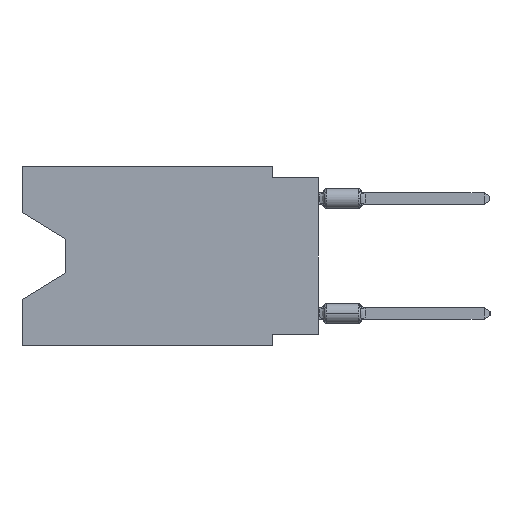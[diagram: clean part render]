
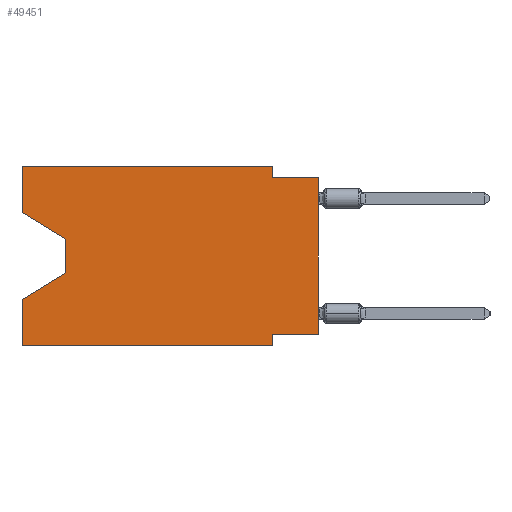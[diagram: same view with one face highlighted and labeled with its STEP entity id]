
A CAD part, left-side view. The second image highlights one B-rep face of the part: STEP entity #49451.
In plain terms, the highlighted planar face has unit normal (-1, 0, 0).
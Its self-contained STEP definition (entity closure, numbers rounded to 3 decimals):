
#1609 = DIRECTION ( 'NONE',  ( 0., -1., 0. ) ) ;
#1917 = LINE ( 'NONE', #22555, #45063 ) ;
#2264 = CARTESIAN_POINT ( 'NONE',  ( 0., 0., -9.271 ) ) ;
#2324 = VECTOR ( 'NONE', #37211, 1000. ) ;
#4034 = CARTESIAN_POINT ( 'NONE',  ( 0., 16.383, 0. ) ) ;
#5596 = VERTEX_POINT ( 'NONE', #2264 ) ;
#6420 = DIRECTION ( 'NONE',  ( 0., 0., -1. ) ) ;
#6921 = EDGE_CURVE ( 'NONE', #15326, #23665, #8161, .T. ) ;
#7123 = LINE ( 'NONE', #8091, #17892 ) ;
#7462 = ORIENTED_EDGE ( 'NONE', *, *, #47942, .T. ) ;
#7670 = EDGE_CURVE ( 'NONE', #15326, #26394, #16879, .T. ) ;
#8091 = CARTESIAN_POINT ( 'NONE',  ( 0., 16.383, -9.906 ) ) ;
#8161 = LINE ( 'NONE', #62636, #9732 ) ;
#8905 = CARTESIAN_POINT ( 'NONE',  ( 0., 16.383, -9.906 ) ) ;
#9318 = CARTESIAN_POINT ( 'NONE',  ( 0., 2.54, 0. ) ) ;
#9732 = VECTOR ( 'NONE', #18971, 1000. ) ;
#10109 = EDGE_CURVE ( 'NONE', #23665, #26422, #49308, .T. ) ;
#11025 = DIRECTION ( 'NONE',  ( 0., -0.855, -0.519 ) ) ;
#11275 = CARTESIAN_POINT ( 'NONE',  ( 0., 16.383, 0. ) ) ;
#11359 = DIRECTION ( 'NONE',  ( 1., 0., 0. ) ) ;
#12468 = LINE ( 'NONE', #52489, #16515 ) ;
#13906 = ORIENTED_EDGE ( 'NONE', *, *, #59940, .T. ) ;
#14040 = ORIENTED_EDGE ( 'NONE', *, *, #25743, .F. ) ;
#15326 = VERTEX_POINT ( 'NONE', #31941 ) ;
#15770 = LINE ( 'NONE', #35784, #16119 ) ;
#16119 = VECTOR ( 'NONE', #24974, 1000. ) ;
#16515 = VECTOR ( 'NONE', #46615, 1000. ) ;
#16879 = LINE ( 'NONE', #40542, #45236 ) ;
#17203 = CARTESIAN_POINT ( 'NONE',  ( 0., 2.54, -9.906 ) ) ;
#17292 = DIRECTION ( 'NONE',  ( 0., -1., 0. ) ) ;
#17892 = VECTOR ( 'NONE', #17292, 1000. ) ;
#18971 = DIRECTION ( 'NONE',  ( 0., 0., 1. ) ) ;
#19718 = CARTESIAN_POINT ( 'NONE',  ( 0., 16.383, -7.36 ) ) ;
#20880 = LINE ( 'NONE', #26137, #31169 ) ;
#21973 = VECTOR ( 'NONE', #61156, 1000. ) ;
#22555 = CARTESIAN_POINT ( 'NONE',  ( 0., 0., -0.635 ) ) ;
#23094 = VERTEX_POINT ( 'NONE', #51480 ) ;
#23176 = CARTESIAN_POINT ( 'NONE',  ( 0., 13.97, -5.893 ) ) ;
#23665 = VERTEX_POINT ( 'NONE', #39142 ) ;
#24304 = LINE ( 'NONE', #44315, #63852 ) ;
#24974 = DIRECTION ( 'NONE',  ( 0., 0., 1. ) ) ;
#25743 = EDGE_CURVE ( 'NONE', #26422, #59305, #33940, .T. ) ;
#26137 = CARTESIAN_POINT ( 'NONE',  ( 0., 0., -9.271 ) ) ;
#26394 = VERTEX_POINT ( 'NONE', #26848 ) ;
#26422 = VERTEX_POINT ( 'NONE', #51790 ) ;
#26746 = ORIENTED_EDGE ( 'NONE', *, *, #46316, .F. ) ;
#26848 = CARTESIAN_POINT ( 'NONE',  ( 0., 13.97, -4.013 ) ) ;
#28974 = DIRECTION ( 'NONE',  ( 0., -1., 0. ) ) ;
#29230 = ORIENTED_EDGE ( 'NONE', *, *, #47190, .F. ) ;
#31169 = VECTOR ( 'NONE', #55033, 1000. ) ;
#31941 = CARTESIAN_POINT ( 'NONE',  ( 0., 16.383, -2.546 ) ) ;
#32000 = CARTESIAN_POINT ( 'NONE',  ( 0., 16.383, 0. ) ) ;
#32278 = EDGE_CURVE ( 'NONE', #49541, #50927, #37526, .T. ) ;
#33044 = ORIENTED_EDGE ( 'NONE', *, *, #55896, .T. ) ;
#33940 = LINE ( 'NONE', #9318, #42179 ) ;
#34199 = EDGE_CURVE ( 'NONE', #5596, #23094, #15770, .T. ) ;
#35784 = CARTESIAN_POINT ( 'NONE',  ( 0., 0., 0. ) ) ;
#36292 = FACE_OUTER_BOUND ( 'NONE', #36623, .T. ) ;
#36623 = EDGE_LOOP ( 'NONE', ( #39455, #13906, #33044, #26746, #7462, #63202, #43557, #44837, #29230, #14040, #46630, #63523 ) ) ;
#37211 = DIRECTION ( 'NONE',  ( 0., 0., -1. ) ) ;
#37526 = LINE ( 'NONE', #17203, #2324 ) ;
#39142 = CARTESIAN_POINT ( 'NONE',  ( 0., 16.383, 0. ) ) ;
#39455 = ORIENTED_EDGE ( 'NONE', *, *, #7670, .T. ) ;
#40542 = CARTESIAN_POINT ( 'NONE',  ( 0., 16.383, -2.546 ) ) ;
#41455 = LINE ( 'NONE', #11275, #21973 ) ;
#42102 = AXIS2_PLACEMENT_3D ( 'NONE', #32000, #11359, #6420 ) ;
#42179 = VECTOR ( 'NONE', #52972, 1000. ) ;
#43557 = ORIENTED_EDGE ( 'NONE', *, *, #57829, .F. ) ;
#44315 = CARTESIAN_POINT ( 'NONE',  ( 0., 13.97, -4.013 ) ) ;
#44837 = ORIENTED_EDGE ( 'NONE', *, *, #34199, .T. ) ;
#45063 = VECTOR ( 'NONE', #1609, 1000. ) ;
#45236 = VECTOR ( 'NONE', #11025, 1000. ) ;
#45421 = CARTESIAN_POINT ( 'NONE',  ( 0., 2.54, -9.906 ) ) ;
#45463 = VERTEX_POINT ( 'NONE', #19718 ) ;
#46080 = VECTOR ( 'NONE', #28974, 1000. ) ;
#46316 = EDGE_CURVE ( 'NONE', #61061, #45463, #41455, .T. ) ;
#46615 = DIRECTION ( 'NONE',  ( 0., 0.855, -0.519 ) ) ;
#46630 = ORIENTED_EDGE ( 'NONE', *, *, #10109, .F. ) ;
#47190 = EDGE_CURVE ( 'NONE', #59305, #23094, #1917, .T. ) ;
#47942 = EDGE_CURVE ( 'NONE', #61061, #50927, #7123, .T. ) ;
#47948 = VERTEX_POINT ( 'NONE', #23176 ) ;
#49308 = LINE ( 'NONE', #4034, #46080 ) ;
#49451 = ADVANCED_FACE ( 'NONE', ( #36292 ), #56309, .F. ) ;
#49541 = VERTEX_POINT ( 'NONE', #52977 ) ;
#50927 = VERTEX_POINT ( 'NONE', #45421 ) ;
#51480 = CARTESIAN_POINT ( 'NONE',  ( 0., 0., -0.635 ) ) ;
#51790 = CARTESIAN_POINT ( 'NONE',  ( 0., 2.54, 0. ) ) ;
#52489 = CARTESIAN_POINT ( 'NONE',  ( 0., 13.97, -5.893 ) ) ;
#52972 = DIRECTION ( 'NONE',  ( 0., 0., -1. ) ) ;
#52977 = CARTESIAN_POINT ( 'NONE',  ( 0., 2.54, -9.271 ) ) ;
#55033 = DIRECTION ( 'NONE',  ( 0., 1., 0. ) ) ;
#55896 = EDGE_CURVE ( 'NONE', #47948, #45463, #12468, .T. ) ;
#56309 = PLANE ( 'NONE',  #42102 ) ;
#57829 = EDGE_CURVE ( 'NONE', #5596, #49541, #20880, .T. ) ;
#58911 = CARTESIAN_POINT ( 'NONE',  ( 0., 2.54, -0.635 ) ) ;
#59305 = VERTEX_POINT ( 'NONE', #58911 ) ;
#59940 = EDGE_CURVE ( 'NONE', #26394, #47948, #24304, .T. ) ;
#61061 = VERTEX_POINT ( 'NONE', #8905 ) ;
#61156 = DIRECTION ( 'NONE',  ( 0., 0., 1. ) ) ;
#62636 = CARTESIAN_POINT ( 'NONE',  ( 0., 16.383, 0. ) ) ;
#63202 = ORIENTED_EDGE ( 'NONE', *, *, #32278, .F. ) ;
#63523 = ORIENTED_EDGE ( 'NONE', *, *, #6921, .F. ) ;
#63852 = VECTOR ( 'NONE', #64343, 1000. ) ;
#64343 = DIRECTION ( 'NONE',  ( 0., 0., -1. ) ) ;
